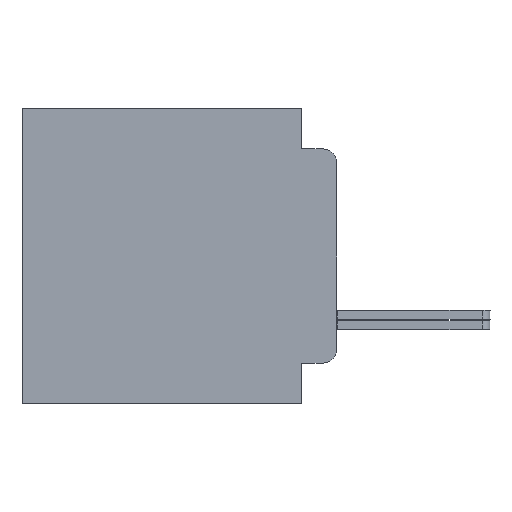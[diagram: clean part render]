
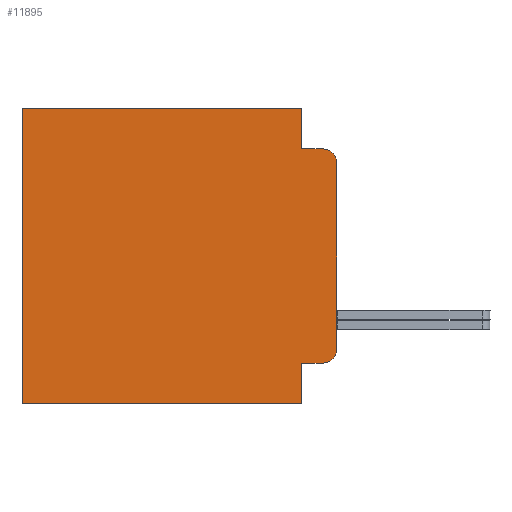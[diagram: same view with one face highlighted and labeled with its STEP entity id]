
A CAD part, left-side view. The second image highlights one B-rep face of the part: STEP entity #11895.
In plain terms, the highlighted planar face has unit normal (-1, 0, 0).
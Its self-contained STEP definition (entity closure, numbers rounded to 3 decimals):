
#108 = CARTESIAN_POINT ( 'NONE',  ( -67.462, 0., 3.467 ) ) ;
#316 = EDGE_CURVE ( 'NONE', #10718, #3792, #25639, .T. ) ;
#327 = VECTOR ( 'NONE', #25184, 1000. ) ;
#562 = ORIENTED_EDGE ( 'NONE', *, *, #11422, .T. ) ;
#846 = ORIENTED_EDGE ( 'NONE', *, *, #8770, .T. ) ;
#1215 = VECTOR ( 'NONE', #23417, 1000. ) ;
#1756 = VERTEX_POINT ( 'NONE', #108 ) ;
#2073 = LINE ( 'NONE', #5353, #14959 ) ;
#2665 = CARTESIAN_POINT ( 'NONE',  ( -67.462, 0., -5.486 ) ) ;
#2774 = EDGE_CURVE ( 'NONE', #25548, #23268, #2073, .T. ) ;
#2965 = LINE ( 'NONE', #22965, #327 ) ;
#3792 = VERTEX_POINT ( 'NONE', #16314 ) ;
#4322 = CARTESIAN_POINT ( 'NONE',  ( -67.462, 0., 5.486 ) ) ;
#4496 = AXIS2_PLACEMENT_3D ( 'NONE', #2665, #17683, #9051 ) ;
#4957 = AXIS2_PLACEMENT_3D ( 'NONE', #18580, #20698, #22352 ) ;
#5222 = CARTESIAN_POINT ( 'NONE',  ( -67.462, 1.295, 0. ) ) ;
#5237 = VERTEX_POINT ( 'NONE', #10509 ) ;
#5263 = ORIENTED_EDGE ( 'NONE', *, *, #7788, .F. ) ;
#5353 = CARTESIAN_POINT ( 'NONE',  ( -67.462, 1.295, -3.975 ) ) ;
#6600 = VECTOR ( 'NONE', #7011, 1000. ) ;
#6649 = EDGE_CURVE ( 'NONE', #23268, #5237, #9062, .T. ) ;
#6874 = EDGE_LOOP ( 'NONE', ( #8787, #24941, #25768, #846, #24826, #8608, #10764, #562, #5263, #14343 ) ) ;
#7011 = DIRECTION ( 'NONE',  ( 0., -1., 0. ) ) ;
#7683 = DIRECTION ( 'NONE',  ( 0., 0., -1. ) ) ;
#7788 = EDGE_CURVE ( 'NONE', #12965, #17522, #21513, .T. ) ;
#8608 = ORIENTED_EDGE ( 'NONE', *, *, #10143, .F. ) ;
#8741 = DIRECTION ( 'NONE',  ( 0., 0., -1. ) ) ;
#8770 = EDGE_CURVE ( 'NONE', #1756, #16616, #18845, .T. ) ;
#8787 = ORIENTED_EDGE ( 'NONE', *, *, #2774, .T. ) ;
#9051 = DIRECTION ( 'NONE',  ( 0., 0., -1. ) ) ;
#9062 = CIRCLE ( 'NONE', #4957, 0.508 ) ;
#9374 = DIRECTION ( 'NONE',  ( 0., -1., 0. ) ) ;
#9845 = CARTESIAN_POINT ( 'NONE',  ( -67.462, 1.295, 5.486 ) ) ;
#9965 = CARTESIAN_POINT ( 'NONE',  ( -67.462, 1.295, -5.486 ) ) ;
#9982 = DIRECTION ( 'NONE',  ( 0., 1., 0. ) ) ;
#10143 = EDGE_CURVE ( 'NONE', #10718, #22854, #23698, .T. ) ;
#10509 = CARTESIAN_POINT ( 'NONE',  ( -67.462, 0., -3.467 ) ) ;
#10718 = VERTEX_POINT ( 'NONE', #9845 ) ;
#10764 = ORIENTED_EDGE ( 'NONE', *, *, #316, .T. ) ;
#11300 = VECTOR ( 'NONE', #7683, 1000. ) ;
#11422 = EDGE_CURVE ( 'NONE', #3792, #17522, #16531, .T. ) ;
#11866 = EDGE_CURVE ( 'NONE', #22854, #16616, #19470, .T. ) ;
#11895 = ADVANCED_FACE ( 'NONE', ( #17161 ), #15503, .F. ) ;
#12191 = CARTESIAN_POINT ( 'NONE',  ( -67.462, 1.295, 3.975 ) ) ;
#12747 = CARTESIAN_POINT ( 'NONE',  ( -67.462, 0.508, 3.467 ) ) ;
#12965 = VERTEX_POINT ( 'NONE', #9965 ) ;
#14049 = AXIS2_PLACEMENT_3D ( 'NONE', #12747, #19116, #8741 ) ;
#14156 = CARTESIAN_POINT ( 'NONE',  ( -67.462, 0., -5.486 ) ) ;
#14343 = ORIENTED_EDGE ( 'NONE', *, *, #19343, .F. ) ;
#14503 = VECTOR ( 'NONE', #25987, 1000. ) ;
#14806 = VECTOR ( 'NONE', #23299, 1000. ) ;
#14959 = VECTOR ( 'NONE', #9374, 1000. ) ;
#15503 = PLANE ( 'NONE',  #4496 ) ;
#16314 = CARTESIAN_POINT ( 'NONE',  ( -67.462, 11.684, 5.486 ) ) ;
#16531 = LINE ( 'NONE', #18263, #11300 ) ;
#16616 = VERTEX_POINT ( 'NONE', #18184 ) ;
#16790 = EDGE_CURVE ( 'NONE', #1756, #5237, #2965, .T. ) ;
#17161 = FACE_OUTER_BOUND ( 'NONE', #6874, .T. ) ;
#17325 = CARTESIAN_POINT ( 'NONE',  ( -67.462, 1.295, 3.975 ) ) ;
#17522 = VERTEX_POINT ( 'NONE', #25427 ) ;
#17683 = DIRECTION ( 'NONE',  ( 1., 0., 0. ) ) ;
#18184 = CARTESIAN_POINT ( 'NONE',  ( -67.462, 0.508, 3.975 ) ) ;
#18263 = CARTESIAN_POINT ( 'NONE',  ( -67.462, 11.684, -5.486 ) ) ;
#18580 = CARTESIAN_POINT ( 'NONE',  ( -67.462, 0.508, -3.467 ) ) ;
#18845 = CIRCLE ( 'NONE', #14049, 0.508 ) ;
#19116 = DIRECTION ( 'NONE',  ( -1., 0., 0. ) ) ;
#19272 = CARTESIAN_POINT ( 'NONE',  ( -67.462, 1.295, -3.975 ) ) ;
#19343 = EDGE_CURVE ( 'NONE', #25548, #12965, #24015, .T. ) ;
#19470 = LINE ( 'NONE', #17325, #6600 ) ;
#20540 = VECTOR ( 'NONE', #9982, 1000. ) ;
#20698 = DIRECTION ( 'NONE',  ( -1., 0., 0. ) ) ;
#21513 = LINE ( 'NONE', #14156, #20540 ) ;
#22352 = DIRECTION ( 'NONE',  ( 0., 0., -1. ) ) ;
#22854 = VERTEX_POINT ( 'NONE', #12191 ) ;
#22965 = CARTESIAN_POINT ( 'NONE',  ( -67.462, 0., -5.486 ) ) ;
#23268 = VERTEX_POINT ( 'NONE', #25865 ) ;
#23299 = DIRECTION ( 'NONE',  ( 0., 0., -1. ) ) ;
#23417 = DIRECTION ( 'NONE',  ( 0., 1., 0. ) ) ;
#23698 = LINE ( 'NONE', #5222, #14503 ) ;
#24015 = LINE ( 'NONE', #25519, #14806 ) ;
#24826 = ORIENTED_EDGE ( 'NONE', *, *, #11866, .F. ) ;
#24941 = ORIENTED_EDGE ( 'NONE', *, *, #6649, .T. ) ;
#25184 = DIRECTION ( 'NONE',  ( 0., 0., -1. ) ) ;
#25427 = CARTESIAN_POINT ( 'NONE',  ( -67.462, 11.684, -5.486 ) ) ;
#25519 = CARTESIAN_POINT ( 'NONE',  ( -67.462, 1.295, 0. ) ) ;
#25548 = VERTEX_POINT ( 'NONE', #19272 ) ;
#25639 = LINE ( 'NONE', #4322, #1215 ) ;
#25768 = ORIENTED_EDGE ( 'NONE', *, *, #16790, .F. ) ;
#25865 = CARTESIAN_POINT ( 'NONE',  ( -67.462, 0.508, -3.975 ) ) ;
#25987 = DIRECTION ( 'NONE',  ( 0., 0., -1. ) ) ;
